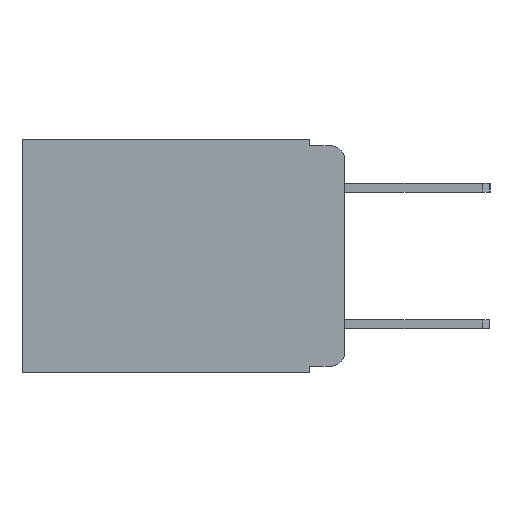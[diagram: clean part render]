
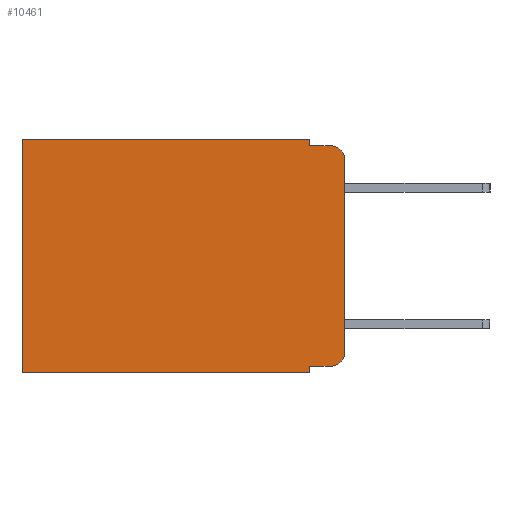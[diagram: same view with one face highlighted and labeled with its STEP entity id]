
A CAD part, left-side view. The second image highlights one B-rep face of the part: STEP entity #10461.
In plain terms, the highlighted planar face has unit normal (-1, 0, 0).
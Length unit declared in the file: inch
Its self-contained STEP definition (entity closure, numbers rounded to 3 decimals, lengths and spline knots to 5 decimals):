
#121 = DIRECTION ( 'NONE',  ( 0., 0., -1. ) ) ;
#442 = DIRECTION ( 'NONE',  ( 0., 0., -1. ) ) ;
#505 = DIRECTION ( 'NONE',  ( -1., 0., 0. ) ) ;
#745 = EDGE_CURVE ( 'NONE', #3052, #1351, #3195, .T. ) ;
#756 = DIRECTION ( 'NONE',  ( 0., 1., 0. ) ) ;
#964 = LINE ( 'NONE', #14859, #14082 ) ;
#1114 = EDGE_LOOP ( 'NONE', ( #10253, #8613, #2147, #8204, #9645, #1682, #1141, #2555, #6770, #8937 ) ) ;
#1141 = ORIENTED_EDGE ( 'NONE', *, *, #4526, .F. ) ;
#1351 = VERTEX_POINT ( 'NONE', #14604 ) ;
#1682 = ORIENTED_EDGE ( 'NONE', *, *, #11950, .T. ) ;
#2002 = LINE ( 'NONE', #14112, #11484 ) ;
#2147 = ORIENTED_EDGE ( 'NONE', *, *, #15037, .F. ) ;
#2175 = EDGE_CURVE ( 'NONE', #15077, #10692, #10818, .T. ) ;
#2555 = ORIENTED_EDGE ( 'NONE', *, *, #11175, .F. ) ;
#3005 = CARTESIAN_POINT ( 'NONE',  ( 0.298, 0.051, 0. ) ) ;
#3045 = DIRECTION ( 'NONE',  ( -1., 0., 0. ) ) ;
#3052 = VERTEX_POINT ( 'NONE', #10035 ) ;
#3195 = CIRCLE ( 'NONE', #5334, 0.02 ) ;
#3234 = VERTEX_POINT ( 'NONE', #7439 ) ;
#3490 = EDGE_CURVE ( 'NONE', #3052, #3234, #13552, .T. ) ;
#3608 = VERTEX_POINT ( 'NONE', #4063 ) ;
#4007 = VERTEX_POINT ( 'NONE', #4573 ) ;
#4063 = CARTESIAN_POINT ( 'NONE',  ( 0.298, 0.051, -0.343 ) ) ;
#4526 = EDGE_CURVE ( 'NONE', #3608, #14862, #2002, .T. ) ;
#4573 = CARTESIAN_POINT ( 'NONE',  ( 0.298, 0.02, -0.333 ) ) ;
#4687 = CARTESIAN_POINT ( 'NONE',  ( 0.298, 0., 0. ) ) ;
#4710 = VECTOR ( 'NONE', #8774, 39.37008 ) ;
#4787 = VECTOR ( 'NONE', #5240, 39.37008 ) ;
#4998 = CARTESIAN_POINT ( 'NONE',  ( 0.298, 0.051, 0. ) ) ;
#5165 = LINE ( 'NONE', #11678, #11266 ) ;
#5240 = DIRECTION ( 'NONE',  ( 0., 0., -1. ) ) ;
#5292 = CARTESIAN_POINT ( 'NONE',  ( 0.298, 0.051, 0. ) ) ;
#5298 = CARTESIAN_POINT ( 'NONE',  ( 0.298, 0.02, -0.03 ) ) ;
#5334 = AXIS2_PLACEMENT_3D ( 'NONE', #5298, #3045, #442 ) ;
#5975 = VECTOR ( 'NONE', #11831, 39.37008 ) ;
#6557 = AXIS2_PLACEMENT_3D ( 'NONE', #14424, #7259, #15554 ) ;
#6770 = ORIENTED_EDGE ( 'NONE', *, *, #10362, .T. ) ;
#7149 = LINE ( 'NONE', #4998, #13563 ) ;
#7259 = DIRECTION ( 'NONE',  ( 1., 0., 0. ) ) ;
#7439 = CARTESIAN_POINT ( 'NONE',  ( 0.298, 0., -0.313 ) ) ;
#7737 = DIRECTION ( 'NONE',  ( 0., -1., 0. ) ) ;
#8149 = CARTESIAN_POINT ( 'NONE',  ( 0.298, 0.02, -0.313 ) ) ;
#8204 = ORIENTED_EDGE ( 'NONE', *, *, #14296, .F. ) ;
#8475 = CIRCLE ( 'NONE', #13194, 0.02 ) ;
#8613 = ORIENTED_EDGE ( 'NONE', *, *, #745, .T. ) ;
#8614 = CARTESIAN_POINT ( 'NONE',  ( 0.298, 0.473, -0.343 ) ) ;
#8774 = DIRECTION ( 'NONE',  ( 0., 1., 0. ) ) ;
#8805 = CARTESIAN_POINT ( 'NONE',  ( 0.298, 0., 0. ) ) ;
#8937 = ORIENTED_EDGE ( 'NONE', *, *, #9528, .T. ) ;
#9041 = CARTESIAN_POINT ( 'NONE',  ( 0.298, 0.473, 0. ) ) ;
#9202 = LINE ( 'NONE', #5292, #4787 ) ;
#9227 = LINE ( 'NONE', #9423, #5975 ) ;
#9316 = DIRECTION ( 'NONE',  ( 0., 0., -1. ) ) ;
#9397 = DIRECTION ( 'NONE',  ( 0., 0., -1. ) ) ;
#9423 = CARTESIAN_POINT ( 'NONE',  ( 0.298, 0.051, -0.333 ) ) ;
#9528 = EDGE_CURVE ( 'NONE', #4007, #3234, #8475, .T. ) ;
#9645 = ORIENTED_EDGE ( 'NONE', *, *, #2175, .T. ) ;
#10005 = DIRECTION ( 'NONE',  ( 0., 0., -1. ) ) ;
#10035 = CARTESIAN_POINT ( 'NONE',  ( 0.298, 0., -0.03 ) ) ;
#10253 = ORIENTED_EDGE ( 'NONE', *, *, #3490, .F. ) ;
#10362 = EDGE_CURVE ( 'NONE', #11318, #4007, #9227, .T. ) ;
#10452 = CARTESIAN_POINT ( 'NONE',  ( 0.298, 0.051, -0.333 ) ) ;
#10461 = ADVANCED_FACE ( 'NONE', ( #13321 ), #13273, .F. ) ;
#10692 = VERTEX_POINT ( 'NONE', #9041 ) ;
#10818 = LINE ( 'NONE', #8805, #4710 ) ;
#11175 = EDGE_CURVE ( 'NONE', #11318, #3608, #9202, .T. ) ;
#11266 = VECTOR ( 'NONE', #9316, 39.37008 ) ;
#11318 = VERTEX_POINT ( 'NONE', #10452 ) ;
#11484 = VECTOR ( 'NONE', #756, 39.37008 ) ;
#11678 = CARTESIAN_POINT ( 'NONE',  ( 0.298, 0.473, 0. ) ) ;
#11831 = DIRECTION ( 'NONE',  ( 0., -1., 0. ) ) ;
#11870 = CARTESIAN_POINT ( 'NONE',  ( 0.298, 0.051, -0.01 ) ) ;
#11950 = EDGE_CURVE ( 'NONE', #10692, #14862, #5165, .T. ) ;
#13194 = AXIS2_PLACEMENT_3D ( 'NONE', #8149, #505, #9397 ) ;
#13273 = PLANE ( 'NONE',  #6557 ) ;
#13292 = VERTEX_POINT ( 'NONE', #11870 ) ;
#13321 = FACE_OUTER_BOUND ( 'NONE', #1114, .T. ) ;
#13552 = LINE ( 'NONE', #4687, #13910 ) ;
#13563 = VECTOR ( 'NONE', #10005, 39.37008 ) ;
#13910 = VECTOR ( 'NONE', #121, 39.37008 ) ;
#14082 = VECTOR ( 'NONE', #7737, 39.37008 ) ;
#14112 = CARTESIAN_POINT ( 'NONE',  ( 0.298, 0., -0.343 ) ) ;
#14296 = EDGE_CURVE ( 'NONE', #15077, #13292, #7149, .T. ) ;
#14424 = CARTESIAN_POINT ( 'NONE',  ( 0.298, 0., 0. ) ) ;
#14604 = CARTESIAN_POINT ( 'NONE',  ( 0.298, 0.02, -0.01 ) ) ;
#14859 = CARTESIAN_POINT ( 'NONE',  ( 0.298, 0.051, -0.01 ) ) ;
#14862 = VERTEX_POINT ( 'NONE', #8614 ) ;
#15037 = EDGE_CURVE ( 'NONE', #13292, #1351, #964, .T. ) ;
#15077 = VERTEX_POINT ( 'NONE', #3005 ) ;
#15554 = DIRECTION ( 'NONE',  ( 0., 0., -1. ) ) ;
